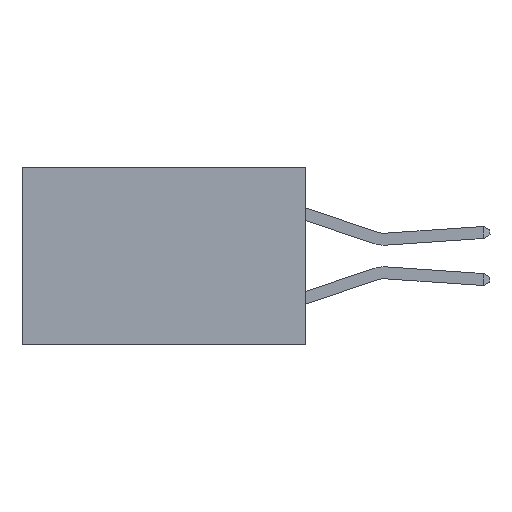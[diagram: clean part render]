
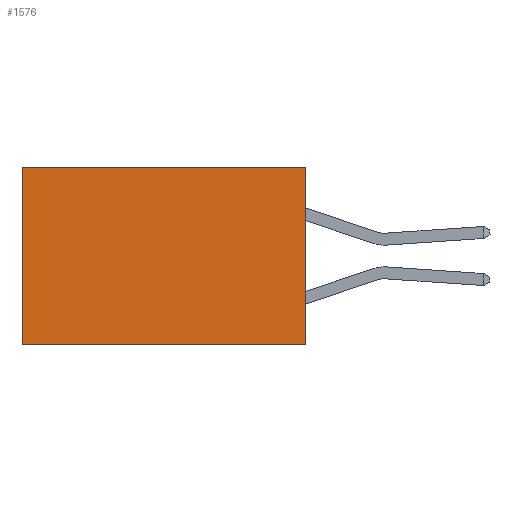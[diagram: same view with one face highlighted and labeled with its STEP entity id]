
A CAD part, left-side view. The second image highlights one B-rep face of the part: STEP entity #1576.
In plain terms, the highlighted planar face has unit normal (-1, 0, 0).
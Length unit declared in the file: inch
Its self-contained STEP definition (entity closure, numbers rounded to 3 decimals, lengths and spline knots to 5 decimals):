
#434 = EDGE_LOOP ( 'NONE', ( #6391, #6597, #3082, #3776 ) ) ;
#536 = VECTOR ( 'NONE', #4100, 39.37008 ) ;
#592 = CARTESIAN_POINT ( 'NONE',  ( 0.277, 0., -0.37 ) ) ;
#909 = CARTESIAN_POINT ( 'NONE',  ( 0.277, 0., 0. ) ) ;
#1179 = CARTESIAN_POINT ( 'NONE',  ( 0.277, 0., -0.37 ) ) ;
#1227 = DIRECTION ( 'NONE',  ( 0., 1., 0. ) ) ;
#1286 = LINE ( 'NONE', #1179, #7067 ) ;
#1576 = ADVANCED_FACE ( 'NONE', ( #4640 ), #2915, .F. ) ;
#1584 = EDGE_CURVE ( 'NONE', #2051, #6068, #2299, .T. ) ;
#1817 = EDGE_CURVE ( 'NONE', #2051, #2040, #8402, .T. ) ;
#2040 = VERTEX_POINT ( 'NONE', #6545 ) ;
#2051 = VERTEX_POINT ( 'NONE', #5347 ) ;
#2299 = LINE ( 'NONE', #8209, #9454 ) ;
#2696 = VECTOR ( 'NONE', #3376, 39.37008 ) ;
#2866 = CARTESIAN_POINT ( 'NONE',  ( 0.277, 0., -0.37 ) ) ;
#2915 = PLANE ( 'NONE',  #4030 ) ;
#3082 = ORIENTED_EDGE ( 'NONE', *, *, #1584, .F. ) ;
#3376 = DIRECTION ( 'NONE',  ( 0., 1., 0. ) ) ;
#3728 = CARTESIAN_POINT ( 'NONE',  ( 0.277, 0.59, -0.37 ) ) ;
#3776 = ORIENTED_EDGE ( 'NONE', *, *, #1817, .T. ) ;
#3877 = VERTEX_POINT ( 'NONE', #3728 ) ;
#4030 = AXIS2_PLACEMENT_3D ( 'NONE', #592, #5003, #8521 ) ;
#4100 = DIRECTION ( 'NONE',  ( 0., 0., -1. ) ) ;
#4214 = CARTESIAN_POINT ( 'NONE',  ( 0.277, 0.59, -0.37 ) ) ;
#4640 = FACE_OUTER_BOUND ( 'NONE', #434, .T. ) ;
#5003 = DIRECTION ( 'NONE',  ( 1., 0., 0. ) ) ;
#5347 = CARTESIAN_POINT ( 'NONE',  ( 0.277, 0., 0. ) ) ;
#5781 = EDGE_CURVE ( 'NONE', #2040, #3877, #8483, .T. ) ;
#6068 = VERTEX_POINT ( 'NONE', #2866 ) ;
#6313 = DIRECTION ( 'NONE',  ( 0., 0., -1. ) ) ;
#6391 = ORIENTED_EDGE ( 'NONE', *, *, #5781, .T. ) ;
#6392 = EDGE_CURVE ( 'NONE', #6068, #3877, #1286, .T. ) ;
#6545 = CARTESIAN_POINT ( 'NONE',  ( 0.277, 0.59, 0. ) ) ;
#6597 = ORIENTED_EDGE ( 'NONE', *, *, #6392, .F. ) ;
#7067 = VECTOR ( 'NONE', #1227, 39.37008 ) ;
#8209 = CARTESIAN_POINT ( 'NONE',  ( 0.277, 0., -0.37 ) ) ;
#8402 = LINE ( 'NONE', #909, #2696 ) ;
#8483 = LINE ( 'NONE', #4214, #536 ) ;
#8521 = DIRECTION ( 'NONE',  ( 0., 0., -1. ) ) ;
#9454 = VECTOR ( 'NONE', #6313, 39.37008 ) ;
